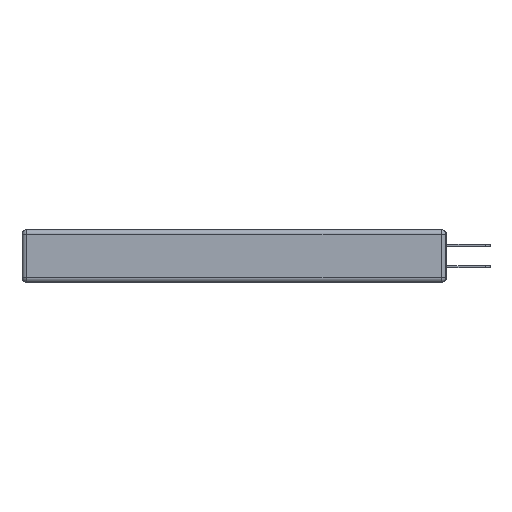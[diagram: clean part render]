
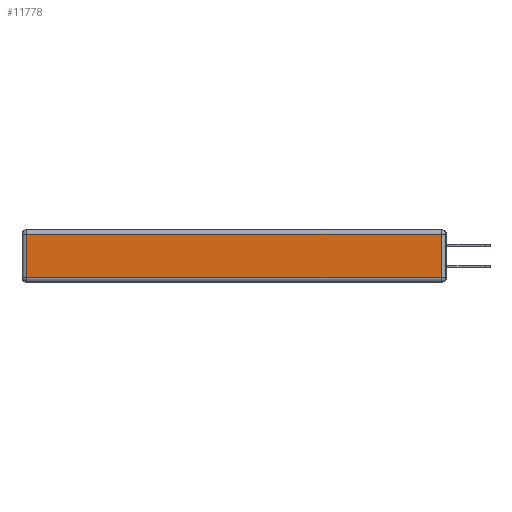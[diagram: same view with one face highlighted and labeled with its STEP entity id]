
A CAD part, left-side view. The second image highlights one B-rep face of the part: STEP entity #11778.
In plain terms, the highlighted planar face has unit normal (-1, 0, 0).
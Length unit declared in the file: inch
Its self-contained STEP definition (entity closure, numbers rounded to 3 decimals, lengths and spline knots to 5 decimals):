
#145 = DIRECTION ( 'NONE',  ( -1., 0., 0. ) ) ;
#2103 = DIRECTION ( 'NONE',  ( 0., 0., -1. ) ) ;
#3176 = CARTESIAN_POINT ( 'NONE',  ( 0., 2.72, -0.313 ) ) ;
#4099 = ORIENTED_EDGE ( 'NONE', *, *, #16386, .T. ) ;
#4391 = ORIENTED_EDGE ( 'NONE', *, *, #14706, .T. ) ;
#5138 = CARTESIAN_POINT ( 'NONE',  ( 0., 2.72, -0.03 ) ) ;
#5198 = DIRECTION ( 'NONE',  ( 0., 0., 1. ) ) ;
#6738 = PLANE ( 'NONE',  #8046 ) ;
#7201 = EDGE_LOOP ( 'NONE', ( #18741, #4099, #14009, #4391 ) ) ;
#8046 = AXIS2_PLACEMENT_3D ( 'NONE', #8443, #145, #5198 ) ;
#8422 = CARTESIAN_POINT ( 'NONE',  ( 0., 0.03, -0.313 ) ) ;
#8443 = CARTESIAN_POINT ( 'NONE',  ( 0., 0., -0.343 ) ) ;
#9433 = DIRECTION ( 'NONE',  ( 0., 1., 0. ) ) ;
#10490 = LINE ( 'NONE', #19844, #17701 ) ;
#11720 = DIRECTION ( 'NONE',  ( 0., -1., 0. ) ) ;
#11778 = ADVANCED_FACE ( 'NONE', ( #13172 ), #6738, .T. ) ;
#12508 = CARTESIAN_POINT ( 'NONE',  ( 0., 0.03, -0.343 ) ) ;
#12629 = VERTEX_POINT ( 'NONE', #8422 ) ;
#13172 = FACE_OUTER_BOUND ( 'NONE', #7201, .T. ) ;
#13298 = LINE ( 'NONE', #12508, #17945 ) ;
#13719 = EDGE_CURVE ( 'NONE', #18181, #19231, #20330, .T. ) ;
#14009 = ORIENTED_EDGE ( 'NONE', *, *, #13719, .T. ) ;
#14706 = EDGE_CURVE ( 'NONE', #19231, #16839, #18983, .T. ) ;
#15178 = CARTESIAN_POINT ( 'NONE',  ( 0., 0.03, -0.03 ) ) ;
#16232 = EDGE_CURVE ( 'NONE', #16839, #12629, #10490, .T. ) ;
#16386 = EDGE_CURVE ( 'NONE', #12629, #18181, #13298, .T. ) ;
#16451 = DIRECTION ( 'NONE',  ( 0., 0., 1. ) ) ;
#16839 = VERTEX_POINT ( 'NONE', #3176 ) ;
#16845 = CARTESIAN_POINT ( 'NONE',  ( 0., 2.72, -0.343 ) ) ;
#17701 = VECTOR ( 'NONE', #11720, 39.37008 ) ;
#17702 = VECTOR ( 'NONE', #2103, 39.37008 ) ;
#17945 = VECTOR ( 'NONE', #16451, 39.37008 ) ;
#18181 = VERTEX_POINT ( 'NONE', #15178 ) ;
#18741 = ORIENTED_EDGE ( 'NONE', *, *, #16232, .T. ) ;
#18983 = LINE ( 'NONE', #16845, #17702 ) ;
#19231 = VERTEX_POINT ( 'NONE', #5138 ) ;
#19306 = CARTESIAN_POINT ( 'NONE',  ( 0., 2.75, -0.03 ) ) ;
#19844 = CARTESIAN_POINT ( 'NONE',  ( 0., 0., -0.313 ) ) ;
#20330 = LINE ( 'NONE', #19306, #20840 ) ;
#20840 = VECTOR ( 'NONE', #9433, 39.37008 ) ;
